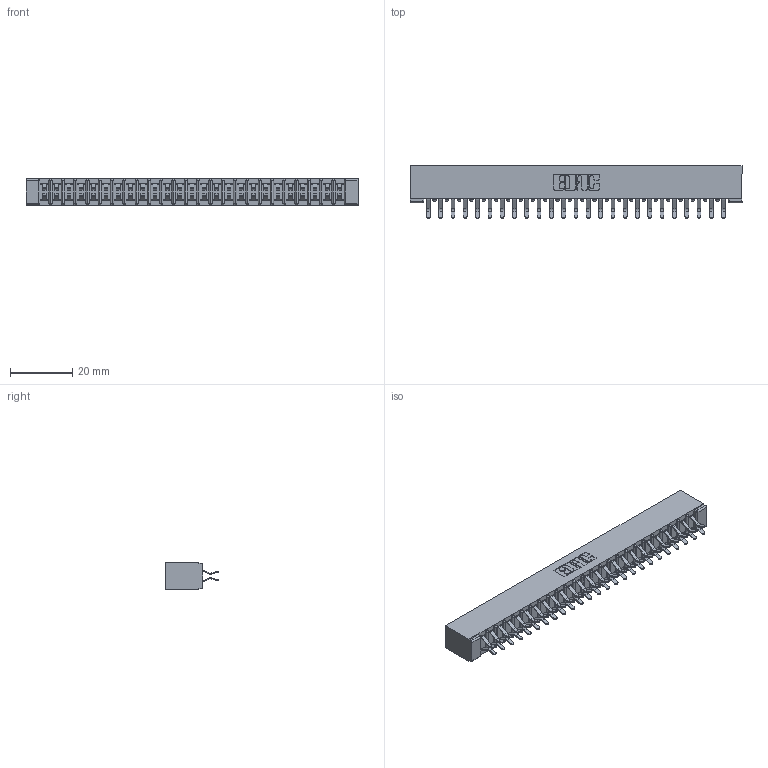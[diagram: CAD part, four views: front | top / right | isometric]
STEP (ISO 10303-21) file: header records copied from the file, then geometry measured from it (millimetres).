
FILE_DESCRIPTION (( 'STEP AP203' ), '1' );
FILE_NAME ('357-050-456-201.STEP', '2020-10-04T05:55:35', ( '' ), ( '' ), 'SwSTEP 2.0', 'SolidWorks 2020', '' );
FILE_SCHEMA (( 'CONFIG_CONTROL_DESIGN' ));
Length unit declared in the file: inch
Products named in the file (3): 307-290-001_556; 357-050-456-201; 307 Part_No Mounting Lugs
Assembly tree (51 placements, depth 2):
  357-050-456-201
    307 Part_No Mounting Lugs
    307-290-001_556  x50
Bounding box: 106.93 x 16.97 x 8.71 mm (x, y, z)
Volume: 7218.3 mm3; surface area: 13326.5 mm2
Topology: 51 solids, 51 shells, 2636 faces, 7399 edges, 4794 vertices
Faces by surface type: plane 1716, cylinder 868, sphere 52
Entity records: 24154 total; most frequent: CARTESIAN_POINT 3953, ORIENTED_EDGE 3914, DIRECTION 3879, EDGE_CURVE 1957, LINE 1495, VECTOR 1495, VERTEX_POINT 1266, AXIS2_PLACEMENT_3D 1192
